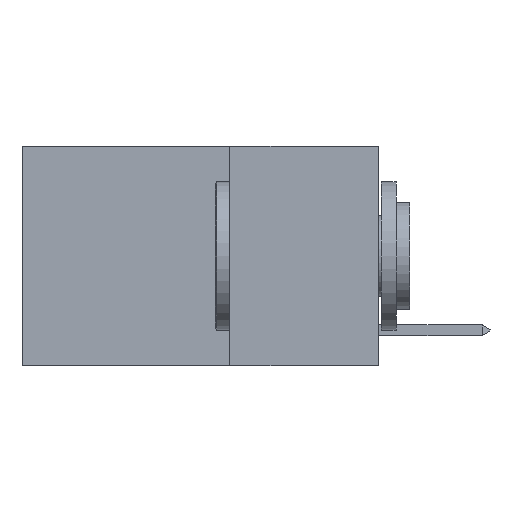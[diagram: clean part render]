
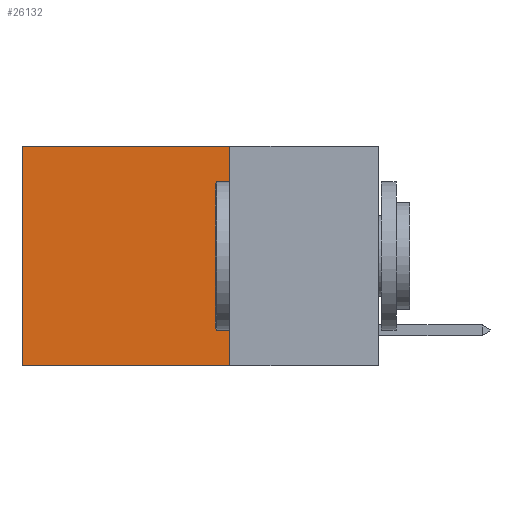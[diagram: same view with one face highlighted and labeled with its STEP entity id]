
A CAD part, left-side view. The second image highlights one B-rep face of the part: STEP entity #26132.
In plain terms, the highlighted planar face has unit normal (-1, 0, 0).
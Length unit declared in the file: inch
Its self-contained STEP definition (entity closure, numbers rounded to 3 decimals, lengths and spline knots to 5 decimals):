
#1415 = ORIENTED_EDGE ( 'NONE', *, *, #10237, .T. ) ;
#1440 = VERTEX_POINT ( 'NONE', #26903 ) ;
#1479 = CARTESIAN_POINT ( 'NONE',  ( 0.2625, 0.6, 0. ) ) ;
#1545 = EDGE_LOOP ( 'NONE', ( #24020, #23376, #8504, #1415 ) ) ;
#2580 = DIRECTION ( 'NONE',  ( 0., 1., 0. ) ) ;
#3869 = DIRECTION ( 'NONE',  ( 0., 0., -1. ) ) ;
#4433 = VERTEX_POINT ( 'NONE', #4889 ) ;
#4889 = CARTESIAN_POINT ( 'NONE',  ( 0.2625, 0.25, 0. ) ) ;
#5296 = LINE ( 'NONE', #1479, #29356 ) ;
#6815 = DIRECTION ( 'NONE',  ( 1., 0., 0. ) ) ;
#8004 = EDGE_CURVE ( 'NONE', #28717, #1440, #17989, .T. ) ;
#8504 = ORIENTED_EDGE ( 'NONE', *, *, #30105, .F. ) ;
#10237 = EDGE_CURVE ( 'NONE', #4433, #13283, #29532, .T. ) ;
#10919 = VECTOR ( 'NONE', #23000, 39.37008 ) ;
#11204 = CARTESIAN_POINT ( 'NONE',  ( 0.2625, 0.25, 0. ) ) ;
#12353 = FACE_OUTER_BOUND ( 'NONE', #1545, .T. ) ;
#13283 = VERTEX_POINT ( 'NONE', #15069 ) ;
#13654 = CARTESIAN_POINT ( 'NONE',  ( 0.2625, 0.25, -0.37 ) ) ;
#15069 = CARTESIAN_POINT ( 'NONE',  ( 0.2625, 0.6, 0. ) ) ;
#16061 = CARTESIAN_POINT ( 'NONE',  ( 0.2625, 0.25, 0. ) ) ;
#16559 = CARTESIAN_POINT ( 'NONE',  ( 0.2625, 0.25, -0.37 ) ) ;
#17832 = VECTOR ( 'NONE', #24693, 39.37008 ) ;
#17989 = LINE ( 'NONE', #16559, #25699 ) ;
#19263 = EDGE_CURVE ( 'NONE', #13283, #1440, #5296, .T. ) ;
#20071 = CARTESIAN_POINT ( 'NONE',  ( 0.2625, 0.25, 0. ) ) ;
#20806 = PLANE ( 'NONE',  #29533 ) ;
#23000 = DIRECTION ( 'NONE',  ( 0., 1., 0. ) ) ;
#23159 = DIRECTION ( 'NONE',  ( 0., 0., -1. ) ) ;
#23376 = ORIENTED_EDGE ( 'NONE', *, *, #8004, .F. ) ;
#24020 = ORIENTED_EDGE ( 'NONE', *, *, #19263, .T. ) ;
#24091 = LINE ( 'NONE', #20071, #17832 ) ;
#24693 = DIRECTION ( 'NONE',  ( 0., 0., -1. ) ) ;
#25699 = VECTOR ( 'NONE', #2580, 39.37008 ) ;
#26132 = ADVANCED_FACE ( 'NONE', ( #12353 ), #20806, .F. ) ;
#26903 = CARTESIAN_POINT ( 'NONE',  ( 0.2625, 0.6, -0.37 ) ) ;
#28717 = VERTEX_POINT ( 'NONE', #13654 ) ;
#29356 = VECTOR ( 'NONE', #3869, 39.37008 ) ;
#29532 = LINE ( 'NONE', #11204, #10919 ) ;
#29533 = AXIS2_PLACEMENT_3D ( 'NONE', #16061, #6815, #23159 ) ;
#30105 = EDGE_CURVE ( 'NONE', #4433, #28717, #24091, .T. ) ;
